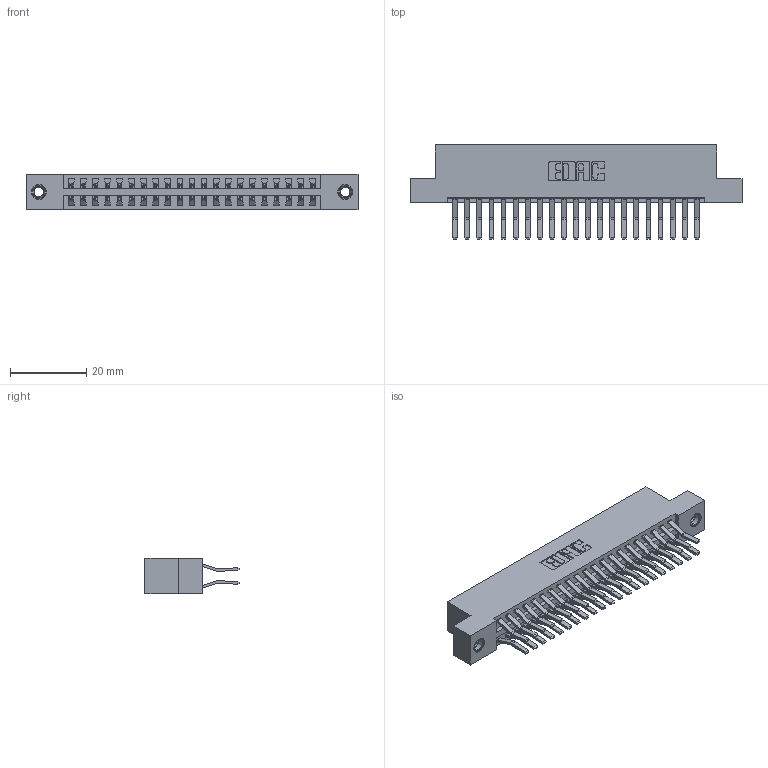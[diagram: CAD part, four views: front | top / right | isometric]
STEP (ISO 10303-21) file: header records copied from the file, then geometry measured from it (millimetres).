
FILE_DESCRIPTION (( 'STEP AP203' ), '1' );
FILE_NAME ('396-042-560-207.STEP', '2018-09-07T01:41:46', ( '' ), ( '' ), 'SwSTEP 2.0', 'SolidWorks 2016', '' );
FILE_SCHEMA (( 'CONFIG_CONTROL_DESIGN' ));
Length unit declared in the file: inch
Products named in the file (4): 346 Part_Flush Mounting Lugs - 0.156 Dia-TI; 345-292-001_560 Tail; 345-250-001_345-250-005-103; 396-042-560-207
Assembly tree (45 placements, depth 2):
  396-042-560-207
    346 Part_Flush Mounting Lugs - 0.156 Dia-TI
    345-292-001_560 Tail  x42
    345-250-001_345-250-005-103  x2
Bounding box: 87.25 x 24.78 x 9.4 mm (x, y, z)
Volume: 8606.5 mm3; surface area: 12268.4 mm2
Topology: 45 solids, 45 shells, 2450 faces, 7227 edges, 4754 vertices
Faces by surface type: plane 1578, cylinder 856, cone 12, torus 4
Entity records: 17806 total; most frequent: CARTESIAN_POINT 2947, ORIENTED_EDGE 2874, DIRECTION 2679, EDGE_CURVE 1437, VECTOR 1197, LINE 1197, VERTEX_POINT 952, AXIS2_PLACEMENT_3D 741
